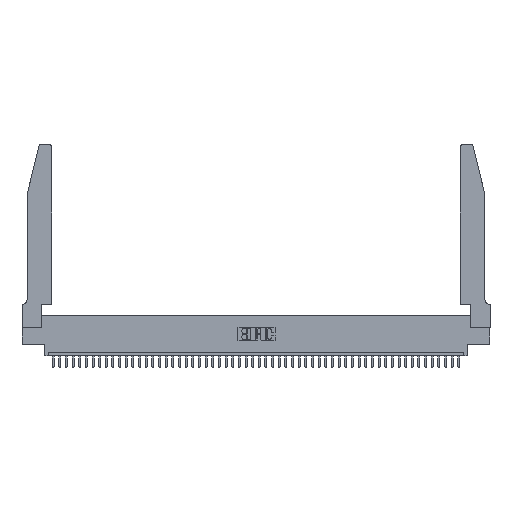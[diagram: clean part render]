
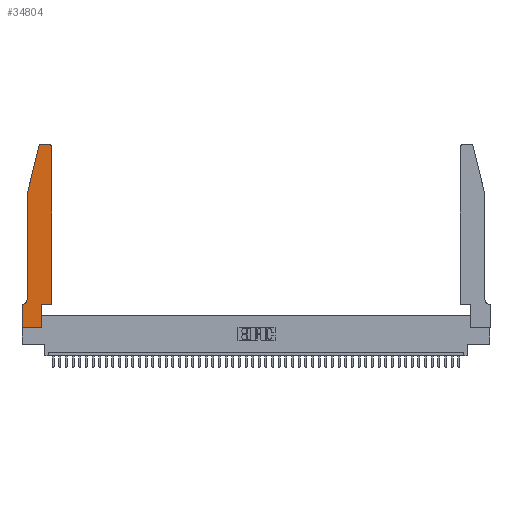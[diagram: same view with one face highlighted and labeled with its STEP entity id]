
A CAD part, top view. The second image highlights one B-rep face of the part: STEP entity #34804.
In plain terms, the highlighted planar face has unit normal (0, 0, 1).
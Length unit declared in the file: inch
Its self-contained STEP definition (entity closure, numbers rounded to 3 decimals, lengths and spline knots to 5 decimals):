
#415 = VECTOR ( 'NONE', #47241, 39.37008 ) ;
#565 = EDGE_CURVE ( 'NONE', #31026, #15763, #26819, .T. ) ;
#1744 = DIRECTION ( 'NONE',  ( 0., 0., 1. ) ) ;
#1842 = VECTOR ( 'NONE', #35519, 39.37008 ) ;
#2004 = ORIENTED_EDGE ( 'NONE', *, *, #29213, .T. ) ;
#2777 = VECTOR ( 'NONE', #44748, 39.37008 ) ;
#4581 = ORIENTED_EDGE ( 'NONE', *, *, #565, .T. ) ;
#4693 = EDGE_CURVE ( 'NONE', #23308, #24978, #43009, .T. ) ;
#5558 = CARTESIAN_POINT ( 'NONE',  ( 0.0755, 2., 0.37 ) ) ;
#5626 = ORIENTED_EDGE ( 'NONE', *, *, #41501, .T. ) ;
#7294 = VECTOR ( 'NONE', #15914, 39.37008 ) ;
#7437 = DIRECTION ( 'NONE',  ( 1., 0., 0. ) ) ;
#9023 = ORIENTED_EDGE ( 'NONE', *, *, #39954, .T. ) ;
#9364 = CARTESIAN_POINT ( 'NONE',  ( 0.0755, 2., 0.37 ) ) ;
#9711 = CARTESIAN_POINT ( 'NONE',  ( 0., 0.35, 0.37 ) ) ;
#10211 = DIRECTION ( 'NONE',  ( 0., 1., 0. ) ) ;
#10646 = LINE ( 'NONE', #32568, #37910 ) ;
#10685 = AXIS2_PLACEMENT_3D ( 'NONE', #18288, #41426, #7437 ) ;
#11512 = FACE_OUTER_BOUND ( 'NONE', #40684, .T. ) ;
#11913 = CARTESIAN_POINT ( 'NONE',  ( 0.4505, 0.35, 0.37 ) ) ;
#12716 = AXIS2_PLACEMENT_3D ( 'NONE', #13981, #40550, #48068 ) ;
#12967 = LINE ( 'NONE', #15150, #46721 ) ;
#13160 = LINE ( 'NONE', #45274, #42223 ) ;
#13216 = ORIENTED_EDGE ( 'NONE', *, *, #4693, .T. ) ;
#13332 = VERTEX_POINT ( 'NONE', #13751 ) ;
#13751 = CARTESIAN_POINT ( 'NONE',  ( 0.284, 2.75, 0.37 ) ) ;
#13981 = CARTESIAN_POINT ( 'NONE',  ( 0.0055, 0.42, 0.37 ) ) ;
#14908 = EDGE_CURVE ( 'NONE', #23179, #13332, #19301, .T. ) ;
#14937 = CARTESIAN_POINT ( 'NONE',  ( 0.2865, 0.35, 0.37 ) ) ;
#15150 = CARTESIAN_POINT ( 'NONE',  ( 0., 0., 0.37 ) ) ;
#15218 = AXIS2_PLACEMENT_3D ( 'NONE', #9711, #1744, #47262 ) ;
#15506 = CARTESIAN_POINT ( 'NONE',  ( 0.4505, 2.72, 0.37 ) ) ;
#15539 = CARTESIAN_POINT ( 'NONE',  ( 0.25487, 2.72718, 0.37 ) ) ;
#15763 = VERTEX_POINT ( 'NONE', #20391 ) ;
#15789 = VERTEX_POINT ( 'NONE', #5558 ) ;
#15914 = DIRECTION ( 'NONE',  ( 1., 0., 0. ) ) ;
#16906 = CARTESIAN_POINT ( 'NONE',  ( 0.2605, 2.75, 0.37 ) ) ;
#18288 = CARTESIAN_POINT ( 'NONE',  ( 0.4205, 2.72, 0.37 ) ) ;
#18521 = EDGE_CURVE ( 'NONE', #48888, #23308, #13160, .T. ) ;
#19004 = LINE ( 'NONE', #9364, #1842 ) ;
#19162 = DIRECTION ( 'NONE',  ( 0., 1., 0. ) ) ;
#19301 = LINE ( 'NONE', #16906, #415 ) ;
#20319 = CIRCLE ( 'NONE', #12716, 0.07 ) ;
#20391 = CARTESIAN_POINT ( 'NONE',  ( 0.2865, 0., 0.37 ) ) ;
#20761 = ORIENTED_EDGE ( 'NONE', *, *, #14908, .T. ) ;
#20862 = ORIENTED_EDGE ( 'NONE', *, *, #30523, .T. ) ;
#21977 = VERTEX_POINT ( 'NONE', #34742 ) ;
#23179 = VERTEX_POINT ( 'NONE', #26224 ) ;
#23308 = VERTEX_POINT ( 'NONE', #11913 ) ;
#23855 = ORIENTED_EDGE ( 'NONE', *, *, #18521, .T. ) ;
#24041 = CARTESIAN_POINT ( 'NONE',  ( 0.0755, 0.42, 0.37 ) ) ;
#24717 = PLANE ( 'NONE',  #15218 ) ;
#24978 = VERTEX_POINT ( 'NONE', #15506 ) ;
#25977 = VECTOR ( 'NONE', #19162, 39.37008 ) ;
#25990 = CARTESIAN_POINT ( 'NONE',  ( 0.0755, 0.35, 0.37 ) ) ;
#26224 = CARTESIAN_POINT ( 'NONE',  ( 0.4205, 2.75, 0.37 ) ) ;
#26819 = LINE ( 'NONE', #34515, #7294 ) ;
#29061 = ORIENTED_EDGE ( 'NONE', *, *, #47616, .T. ) ;
#29213 = EDGE_CURVE ( 'NONE', #15789, #41781, #19004, .T. ) ;
#30523 = EDGE_CURVE ( 'NONE', #37806, #31026, #12967, .T. ) ;
#30601 = EDGE_CURVE ( 'NONE', #15763, #48888, #37318, .T. ) ;
#30813 = DIRECTION ( 'NONE',  ( 0., 0., 1. ) ) ;
#31026 = VERTEX_POINT ( 'NONE', #46371 ) ;
#31552 = CIRCLE ( 'NONE', #10685, 0.03 ) ;
#32568 = CARTESIAN_POINT ( 'NONE',  ( 0.0755, 2., 0.37 ) ) ;
#33735 = CARTESIAN_POINT ( 'NONE',  ( 0.2865, 0.35, 0.37 ) ) ;
#34515 = CARTESIAN_POINT ( 'NONE',  ( 0., 0., 0.37 ) ) ;
#34719 = ORIENTED_EDGE ( 'NONE', *, *, #30601, .T. ) ;
#34742 = CARTESIAN_POINT ( 'NONE',  ( 0.0055, 0.35, 0.37 ) ) ;
#34804 = ADVANCED_FACE ( 'NONE', ( #11512 ), #24717, .T. ) ;
#35308 = LINE ( 'NONE', #25990, #2777 ) ;
#35519 = DIRECTION ( 'NONE',  ( 0., -1., 0. ) ) ;
#37253 = ORIENTED_EDGE ( 'NONE', *, *, #39339, .T. ) ;
#37318 = LINE ( 'NONE', #14937, #25977 ) ;
#37806 = VERTEX_POINT ( 'NONE', #48065 ) ;
#37858 = DIRECTION ( 'NONE',  ( 1., 0., 0. ) ) ;
#37910 = VECTOR ( 'NONE', #48274, 39.37008 ) ;
#39339 = EDGE_CURVE ( 'NONE', #13332, #40179, #44246, .T. ) ;
#39954 = EDGE_CURVE ( 'NONE', #21977, #37806, #35308, .T. ) ;
#40179 = VERTEX_POINT ( 'NONE', #15539 ) ;
#40550 = DIRECTION ( 'NONE',  ( 0., 0., -1. ) ) ;
#40684 = EDGE_LOOP ( 'NONE', ( #20761, #37253, #48973, #2004, #29061, #9023, #20862, #4581, #34719, #23855, #13216, #5626 ) ) ;
#41317 = DIRECTION ( 'NONE',  ( 0., -1., 0. ) ) ;
#41426 = DIRECTION ( 'NONE',  ( 0., 0., 1. ) ) ;
#41501 = EDGE_CURVE ( 'NONE', #24978, #23179, #31552, .T. ) ;
#41724 = AXIS2_PLACEMENT_3D ( 'NONE', #45898, #30813, #45593 ) ;
#41781 = VERTEX_POINT ( 'NONE', #24041 ) ;
#42223 = VECTOR ( 'NONE', #37858, 39.37008 ) ;
#43009 = LINE ( 'NONE', #47749, #44835 ) ;
#44246 = CIRCLE ( 'NONE', #41724, 0.03 ) ;
#44606 = EDGE_CURVE ( 'NONE', #40179, #15789, #10646, .T. ) ;
#44748 = DIRECTION ( 'NONE',  ( -1., 0., 0. ) ) ;
#44835 = VECTOR ( 'NONE', #10211, 39.37008 ) ;
#45274 = CARTESIAN_POINT ( 'NONE',  ( 0.4505, 0.35, 0.37 ) ) ;
#45593 = DIRECTION ( 'NONE',  ( 1., 0., 0. ) ) ;
#45898 = CARTESIAN_POINT ( 'NONE',  ( 0.284, 2.72, 0.37 ) ) ;
#46371 = CARTESIAN_POINT ( 'NONE',  ( 0., 0., 0.37 ) ) ;
#46721 = VECTOR ( 'NONE', #41317, 39.37008 ) ;
#47241 = DIRECTION ( 'NONE',  ( -1., 0., 0. ) ) ;
#47262 = DIRECTION ( 'NONE',  ( 1., 0., 0. ) ) ;
#47616 = EDGE_CURVE ( 'NONE', #41781, #21977, #20319, .T. ) ;
#47749 = CARTESIAN_POINT ( 'NONE',  ( 0.4505, 0.35, 0.37 ) ) ;
#48065 = CARTESIAN_POINT ( 'NONE',  ( 0., 0.35, 0.37 ) ) ;
#48068 = DIRECTION ( 'NONE',  ( -1., 0., 0. ) ) ;
#48274 = DIRECTION ( 'NONE',  ( -0.239, -0.971, 0. ) ) ;
#48888 = VERTEX_POINT ( 'NONE', #33735 ) ;
#48973 = ORIENTED_EDGE ( 'NONE', *, *, #44606, .T. ) ;
